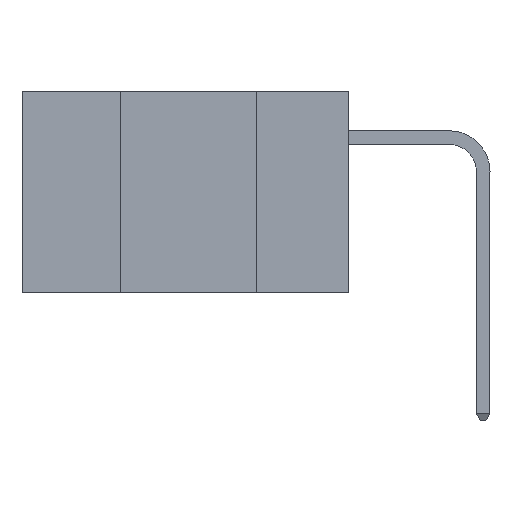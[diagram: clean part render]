
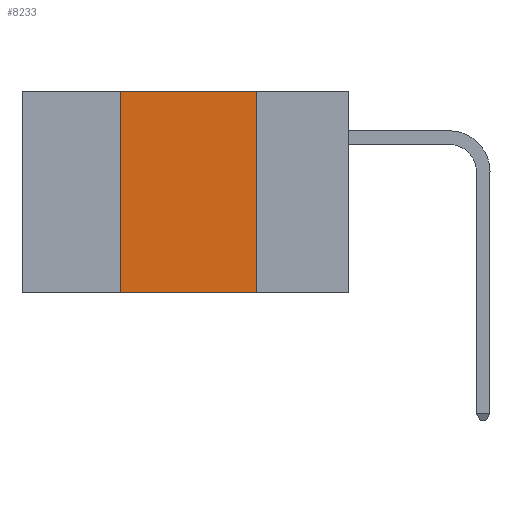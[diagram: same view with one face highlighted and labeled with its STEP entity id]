
A CAD part, left-side view. The second image highlights one B-rep face of the part: STEP entity #8233.
In plain terms, the highlighted planar face has unit normal (-1, 0, 0).
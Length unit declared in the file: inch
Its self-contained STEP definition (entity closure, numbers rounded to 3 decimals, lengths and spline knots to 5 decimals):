
#351 = VERTEX_POINT ( 'NONE', #23469 ) ;
#384 = VERTEX_POINT ( 'NONE', #6729 ) ;
#3159 = ORIENTED_EDGE ( 'NONE', *, *, #15795, .T. ) ;
#3259 = EDGE_CURVE ( 'NONE', #384, #23996, #4647, .T. ) ;
#3783 = ORIENTED_EDGE ( 'NONE', *, *, #3259, .F. ) ;
#4308 = CARTESIAN_POINT ( 'NONE',  ( 0., 0.42, 0. ) ) ;
#4647 = LINE ( 'NONE', #24544, #15227 ) ;
#6068 = CARTESIAN_POINT ( 'NONE',  ( 0., 0.6, -0.37 ) ) ;
#6729 = CARTESIAN_POINT ( 'NONE',  ( 0., 0.42, -0.37 ) ) ;
#6757 = CARTESIAN_POINT ( 'NONE',  ( 0., 0.6, 0. ) ) ;
#7342 = DIRECTION ( 'NONE',  ( 0., -1., 0. ) ) ;
#8233 = ADVANCED_FACE ( 'NONE', ( #16928 ), #23575, .F. ) ;
#8506 = LINE ( 'NONE', #6068, #9828 ) ;
#8510 = LINE ( 'NONE', #15544, #19071 ) ;
#9810 = DIRECTION ( 'NONE',  ( 0., 0., 1. ) ) ;
#9828 = VECTOR ( 'NONE', #10315, 39.37008 ) ;
#10169 = ORIENTED_EDGE ( 'NONE', *, *, #13717, .F. ) ;
#10315 = DIRECTION ( 'NONE',  ( 0., -1., 0. ) ) ;
#10973 = DIRECTION ( 'NONE',  ( 1., 0., 0. ) ) ;
#13717 = EDGE_CURVE ( 'NONE', #23996, #351, #20496, .T. ) ;
#14434 = ORIENTED_EDGE ( 'NONE', *, *, #21151, .F. ) ;
#14834 = VECTOR ( 'NONE', #7342, 39.37008 ) ;
#15227 = VECTOR ( 'NONE', #9810, 39.37008 ) ;
#15544 = CARTESIAN_POINT ( 'NONE',  ( 0., 0.17, 0. ) ) ;
#15569 = VERTEX_POINT ( 'NONE', #22210 ) ;
#15795 = EDGE_CURVE ( 'NONE', #384, #15569, #8506, .T. ) ;
#16928 = FACE_OUTER_BOUND ( 'NONE', #23684, .T. ) ;
#17674 = DIRECTION ( 'NONE',  ( 0., 0., -1. ) ) ;
#18338 = AXIS2_PLACEMENT_3D ( 'NONE', #6757, #10973, #25730 ) ;
#19071 = VECTOR ( 'NONE', #17674, 39.37008 ) ;
#19876 = CARTESIAN_POINT ( 'NONE',  ( 0., 0.6, 0. ) ) ;
#20496 = LINE ( 'NONE', #19876, #14834 ) ;
#21151 = EDGE_CURVE ( 'NONE', #351, #15569, #8510, .T. ) ;
#22210 = CARTESIAN_POINT ( 'NONE',  ( 0., 0.17, -0.37 ) ) ;
#23469 = CARTESIAN_POINT ( 'NONE',  ( 0., 0.17, 0. ) ) ;
#23575 = PLANE ( 'NONE',  #18338 ) ;
#23684 = EDGE_LOOP ( 'NONE', ( #14434, #10169, #3783, #3159 ) ) ;
#23996 = VERTEX_POINT ( 'NONE', #4308 ) ;
#24544 = CARTESIAN_POINT ( 'NONE',  ( 0., 0.42, 0. ) ) ;
#25730 = DIRECTION ( 'NONE',  ( 0., 0., -1. ) ) ;
